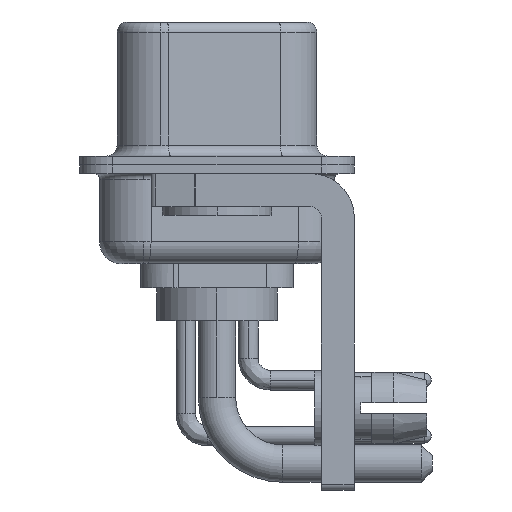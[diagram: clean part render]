
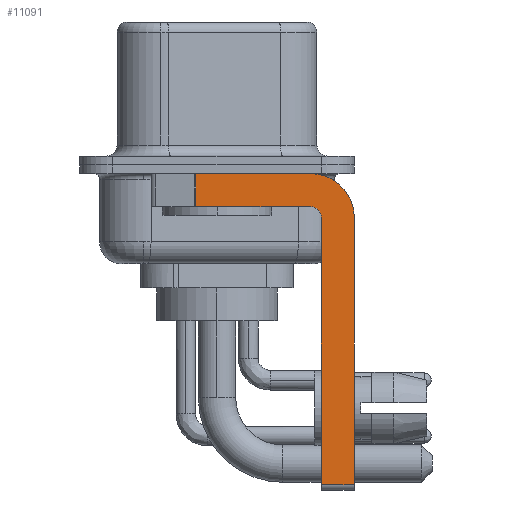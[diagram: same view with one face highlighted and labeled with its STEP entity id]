
A CAD part, left-side view. The second image highlights one B-rep face of the part: STEP entity #11091.
In plain terms, the highlighted planar face has unit normal (-1, 0, 0).
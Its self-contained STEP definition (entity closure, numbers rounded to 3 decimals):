
#1059 = DIRECTION ( 'NONE',  ( 0., 1., 0. ) ) ;
#1160 = DIRECTION ( 'NONE',  ( 0., 0., -1. ) ) ;
#1169 = CARTESIAN_POINT ( 'NONE',  ( -2.9, -4.75, -2.4 ) ) ;
#2227 = EDGE_CURVE ( 'NONE', #10773, #23054, #12310, .T. ) ;
#2255 = CARTESIAN_POINT ( 'NONE',  ( -2.9, 0.978, -1.9 ) ) ;
#2279 = CARTESIAN_POINT ( 'NONE',  ( -2.9, -4.25, -0.4 ) ) ;
#2300 = ORIENTED_EDGE ( 'NONE', *, *, #2572, .F. ) ;
#2480 = AXIS2_PLACEMENT_3D ( 'NONE', #7165, #11390, #2629 ) ;
#2572 = EDGE_CURVE ( 'NONE', #22784, #23054, #16379, .T. ) ;
#2629 = DIRECTION ( 'NONE',  ( 0., 0., 1. ) ) ;
#3369 = DIRECTION ( 'NONE',  ( 0., 0., -1. ) ) ;
#3523 = VECTOR ( 'NONE', #3369, 1000. ) ;
#4196 = ORIENTED_EDGE ( 'NONE', *, *, #13397, .F. ) ;
#4200 = ORIENTED_EDGE ( 'NONE', *, *, #7963, .F. ) ;
#4789 = LINE ( 'NONE', #20038, #16590 ) ;
#5578 = VERTEX_POINT ( 'NONE', #2255 ) ;
#5607 = ORIENTED_EDGE ( 'NONE', *, *, #17615, .F. ) ;
#5880 = DIRECTION ( 'NONE',  ( 0., -1., 0. ) ) ;
#7034 = VECTOR ( 'NONE', #1059, 1000. ) ;
#7165 = CARTESIAN_POINT ( 'NONE',  ( -2.9, -4.25, -2.4 ) ) ;
#7194 = DIRECTION ( 'NONE',  ( 0., 0., 1. ) ) ;
#7320 = DIRECTION ( 'NONE',  ( 0., 0., -1. ) ) ;
#7765 = LINE ( 'NONE', #20197, #3523 ) ;
#7963 = EDGE_CURVE ( 'NONE', #17017, #22547, #27811, .T. ) ;
#8450 = CARTESIAN_POINT ( 'NONE',  ( -2.9, -4.75, -14.55 ) ) ;
#9629 = DIRECTION ( 'NONE',  ( 0., -1., 0. ) ) ;
#9859 = LINE ( 'NONE', #13810, #7034 ) ;
#10105 = VERTEX_POINT ( 'NONE', #2279 ) ;
#10668 = EDGE_CURVE ( 'NONE', #26270, #5578, #7765, .T. ) ;
#10773 = VERTEX_POINT ( 'NONE', #8450 ) ;
#11091 = ADVANCED_FACE ( 'NONE', ( #20846 ), #16604, .F. ) ;
#11390 = DIRECTION ( 'NONE',  ( -1., 0., 0. ) ) ;
#12310 = LINE ( 'NONE', #20940, #26754 ) ;
#12749 = ORIENTED_EDGE ( 'NONE', *, *, #2227, .T. ) ;
#13193 = VECTOR ( 'NONE', #5880, 1000. ) ;
#13397 = EDGE_CURVE ( 'NONE', #10105, #22784, #22100, .T. ) ;
#13810 = CARTESIAN_POINT ( 'NONE',  ( -2.9, -4.25, -1.9 ) ) ;
#14272 = ORIENTED_EDGE ( 'NONE', *, *, #22380, .F. ) ;
#16247 = DIRECTION ( 'NONE',  ( 0., 0., -1. ) ) ;
#16379 = LINE ( 'NONE', #24751, #27712 ) ;
#16590 = VECTOR ( 'NONE', #7194, 1000. ) ;
#16604 = PLANE ( 'NONE',  #22506 ) ;
#16620 = LINE ( 'NONE', #25256, #13193 ) ;
#16919 = ORIENTED_EDGE ( 'NONE', *, *, #20999, .F. ) ;
#17017 = VERTEX_POINT ( 'NONE', #1169 ) ;
#17615 = EDGE_CURVE ( 'NONE', #26270, #10105, #16620, .T. ) ;
#20038 = CARTESIAN_POINT ( 'NONE',  ( -2.9, -4.75, -14.8 ) ) ;
#20197 = CARTESIAN_POINT ( 'NONE',  ( -2.9, 0.978, -1.9 ) ) ;
#20266 = AXIS2_PLACEMENT_3D ( 'NONE', #26439, #26715, #7320 ) ;
#20561 = CARTESIAN_POINT ( 'NONE',  ( -2.9, -4.25, -2.4 ) ) ;
#20846 = FACE_OUTER_BOUND ( 'NONE', #22523, .T. ) ;
#20940 = CARTESIAN_POINT ( 'NONE',  ( -2.9, -4.25, -14.55 ) ) ;
#20999 = EDGE_CURVE ( 'NONE', #22547, #5578, #9859, .T. ) ;
#22100 = CIRCLE ( 'NONE', #20266, 2. ) ;
#22371 = CARTESIAN_POINT ( 'NONE',  ( -2.9, -6.25, -14.55 ) ) ;
#22380 = EDGE_CURVE ( 'NONE', #10773, #17017, #4789, .T. ) ;
#22506 = AXIS2_PLACEMENT_3D ( 'NONE', #20561, #25241, #1160 ) ;
#22523 = EDGE_LOOP ( 'NONE', ( #5607, #25867, #16919, #4200, #14272, #12749, #2300, #4196 ) ) ;
#22547 = VERTEX_POINT ( 'NONE', #27277 ) ;
#22784 = VERTEX_POINT ( 'NONE', #23875 ) ;
#23054 = VERTEX_POINT ( 'NONE', #22371 ) ;
#23875 = CARTESIAN_POINT ( 'NONE',  ( -2.9, -6.25, -2.4 ) ) ;
#24751 = CARTESIAN_POINT ( 'NONE',  ( -2.9, -6.25, -2.4 ) ) ;
#25241 = DIRECTION ( 'NONE',  ( 1., 0., 0. ) ) ;
#25256 = CARTESIAN_POINT ( 'NONE',  ( -2.9, 3., -0.4 ) ) ;
#25867 = ORIENTED_EDGE ( 'NONE', *, *, #10668, .T. ) ;
#26270 = VERTEX_POINT ( 'NONE', #27689 ) ;
#26439 = CARTESIAN_POINT ( 'NONE',  ( -2.9, -4.25, -2.4 ) ) ;
#26715 = DIRECTION ( 'NONE',  ( 1., 0., 0. ) ) ;
#26754 = VECTOR ( 'NONE', #9629, 1000. ) ;
#27277 = CARTESIAN_POINT ( 'NONE',  ( -2.9, -4.25, -1.9 ) ) ;
#27689 = CARTESIAN_POINT ( 'NONE',  ( -2.9, 0.978, -0.4 ) ) ;
#27712 = VECTOR ( 'NONE', #16247, 1000. ) ;
#27811 = CIRCLE ( 'NONE', #2480, 0.5 ) ;
